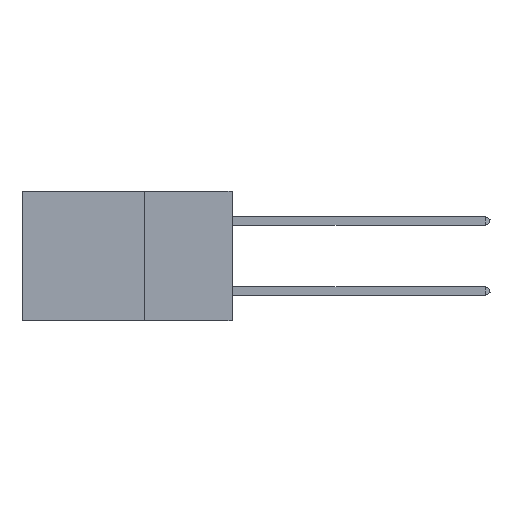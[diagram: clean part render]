
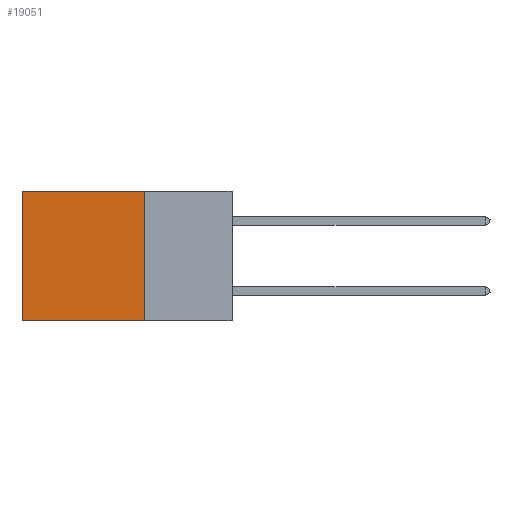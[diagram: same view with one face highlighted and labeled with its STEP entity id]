
A CAD part, left-side view. The second image highlights one B-rep face of the part: STEP entity #19051.
In plain terms, the highlighted planar face has unit normal (-1, 0, 0).
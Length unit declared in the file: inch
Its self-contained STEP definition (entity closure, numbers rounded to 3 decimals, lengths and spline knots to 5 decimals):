
#472 = VECTOR ( 'NONE', #15024, 39.37008 ) ;
#1587 = LINE ( 'NONE', #2885, #472 ) ;
#1746 = AXIS2_PLACEMENT_3D ( 'NONE', #6859, #23364, #30629 ) ;
#2885 = CARTESIAN_POINT ( 'NONE',  ( 0.2875, 0.25, -0.37 ) ) ;
#3734 = VECTOR ( 'NONE', #11400, 39.37008 ) ;
#4388 = CARTESIAN_POINT ( 'NONE',  ( 0.2875, 0.6, -0.37 ) ) ;
#4735 = VERTEX_POINT ( 'NONE', #13256 ) ;
#6322 = VERTEX_POINT ( 'NONE', #21073 ) ;
#6701 = FACE_OUTER_BOUND ( 'NONE', #15199, .T. ) ;
#6859 = CARTESIAN_POINT ( 'NONE',  ( 0.2875, 0.25, 0. ) ) ;
#7295 = VECTOR ( 'NONE', #29049, 39.37008 ) ;
#7555 = VERTEX_POINT ( 'NONE', #4388 ) ;
#7870 = EDGE_CURVE ( 'NONE', #6322, #7555, #1587, .T. ) ;
#9303 = ORIENTED_EDGE ( 'NONE', *, *, #26760, .F. ) ;
#9380 = ORIENTED_EDGE ( 'NONE', *, *, #19515, .T. ) ;
#9882 = CARTESIAN_POINT ( 'NONE',  ( 0.2875, 0.25, 0. ) ) ;
#10039 = LINE ( 'NONE', #23440, #3734 ) ;
#11400 = DIRECTION ( 'NONE',  ( 0., 0., -1. ) ) ;
#12352 = EDGE_CURVE ( 'NONE', #24418, #4735, #16583, .T. ) ;
#12899 = ORIENTED_EDGE ( 'NONE', *, *, #12352, .T. ) ;
#13256 = CARTESIAN_POINT ( 'NONE',  ( 0.2875, 0.6, 0. ) ) ;
#13764 = VECTOR ( 'NONE', #25893, 39.37008 ) ;
#15024 = DIRECTION ( 'NONE',  ( 0., 1., 0. ) ) ;
#15199 = EDGE_LOOP ( 'NONE', ( #9380, #29601, #9303, #12899 ) ) ;
#16583 = LINE ( 'NONE', #9882, #7295 ) ;
#19051 = ADVANCED_FACE ( 'NONE', ( #6701 ), #20901, .F. ) ;
#19515 = EDGE_CURVE ( 'NONE', #4735, #7555, #26390, .T. ) ;
#20826 = CARTESIAN_POINT ( 'NONE',  ( 0.2875, 0.6, 0. ) ) ;
#20901 = PLANE ( 'NONE',  #1746 ) ;
#21073 = CARTESIAN_POINT ( 'NONE',  ( 0.2875, 0.25, -0.37 ) ) ;
#21885 = CARTESIAN_POINT ( 'NONE',  ( 0.2875, 0.25, 0. ) ) ;
#23364 = DIRECTION ( 'NONE',  ( 1., 0., 0. ) ) ;
#23440 = CARTESIAN_POINT ( 'NONE',  ( 0.2875, 0.25, 0. ) ) ;
#24418 = VERTEX_POINT ( 'NONE', #21885 ) ;
#25893 = DIRECTION ( 'NONE',  ( 0., 0., -1. ) ) ;
#26390 = LINE ( 'NONE', #20826, #13764 ) ;
#26760 = EDGE_CURVE ( 'NONE', #24418, #6322, #10039, .T. ) ;
#29049 = DIRECTION ( 'NONE',  ( 0., 1., 0. ) ) ;
#29601 = ORIENTED_EDGE ( 'NONE', *, *, #7870, .F. ) ;
#30629 = DIRECTION ( 'NONE',  ( 0., 0., -1. ) ) ;
